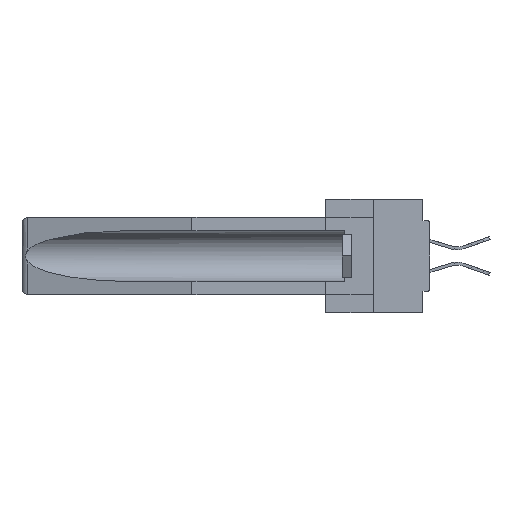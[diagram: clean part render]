
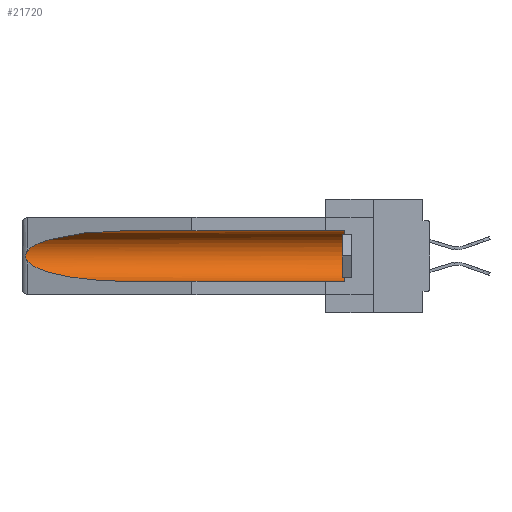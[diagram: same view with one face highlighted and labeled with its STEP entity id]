
A CAD part, left-side view. The second image highlights one B-rep face of the part: STEP entity #21720.
In plain terms, the highlighted cylindrical face has radius 2.857 mm (diameter 5.715 mm), a partial arc.
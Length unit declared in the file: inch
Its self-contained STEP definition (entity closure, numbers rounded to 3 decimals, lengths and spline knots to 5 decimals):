
#27 = EDGE_CURVE ( 'NONE', #23490, #26655, #21769, .T. ) ;
#66 = CARTESIAN_POINT ( 'NONE',  ( 0.2675, 1.53308, -0.16763 ) ) ;
#381 = EDGE_LOOP ( 'NONE', ( #35002, #39673, #11307, #32883, #12412, #17191 ) ) ;
#655 = EDGE_CURVE ( 'NONE', #15124, #21723, #30816, .T. ) ;
#1708 = AXIS2_PLACEMENT_3D ( 'NONE', #29008, #10646, #13699 ) ;
#2555 = CARTESIAN_POINT ( 'NONE',  ( 0.155, -0.30754, -0.059 ) ) ;
#6058 = CARTESIAN_POINT ( 'NONE',  ( 0.26654, 1.53092, -0.15636 ) ) ;
#8360 = CARTESIAN_POINT ( 'NONE',  ( 0.155, 0.126, -0.1715 ) ) ;
#8729 = CARTESIAN_POINT ( 'NONE',  ( 0.26537, 1.52718, -0.19328 ) ) ;
#8858 = CARTESIAN_POINT ( 'NONE',  ( 0.26597, 1.5296, -0.19026 ) ) ;
#8891 = CARTESIAN_POINT ( 'NONE',  ( 0.26537, 1.52718, -0.14972 ) ) ;
#9084 = VECTOR ( 'NONE', #39557, 39.37008 ) ;
#9232 = CARTESIAN_POINT ( 'NONE',  ( 0.21114, 1.30732, -0.059 ) ) ;
#10646 = DIRECTION ( 'NONE',  ( 0., 1., 0. ) ) ;
#11240 = VERTEX_POINT ( 'NONE', #8891 ) ;
#11307 = ORIENTED_EDGE ( 'NONE', *, *, #27, .T. ) ;
#12412 = ORIENTED_EDGE ( 'NONE', *, *, #655, .T. ) ;
#13699 = DIRECTION ( 'NONE',  ( 0., 0., 1. ) ) ;
#14834 = LINE ( 'NONE', #2555, #9084 ) ;
#15124 = VERTEX_POINT ( 'NONE', #22785 ) ;
#15191 = CARTESIAN_POINT ( 'NONE',  ( 0.25451, 1.48313, -0.24835 ) ) ;
#15250 = CARTESIAN_POINT ( 'NONE',  ( 0.26537, 1.52718, -0.19328 ) ) ;
#15531 = EDGE_CURVE ( 'NONE', #38226, #11240, #17136, .T. ) ;
#16659 = LINE ( 'NONE', #20119, #23309 ) ;
#17136 =( BOUNDED_CURVE ( )  B_SPLINE_CURVE ( 3, ( #36524, #9232, #37329, #37182 ),
 .UNSPECIFIED., .F., .F. ) 
 B_SPLINE_CURVE_WITH_KNOTS ( ( 4, 4 ),
 ( 4.71239, 6.08839 ),
 .UNSPECIFIED. ) 
 CURVE ( )  GEOMETRIC_REPRESENTATION_ITEM ( )  RATIONAL_B_SPLINE_CURVE ( ( 1., 0.848, 0.848, 1. ) ) 
 REPRESENTATION_ITEM ( '' )  );
#17191 = ORIENTED_EDGE ( 'NONE', *, *, #30240, .T. ) ;
#19035 = AXIS2_PLACEMENT_3D ( 'NONE', #8360, #28179, #21498 ) ;
#19259 = B_SPLINE_CURVE_WITH_KNOTS ( 'NONE', 3,
 ( #27321, #24142, #6058, #33700, #66, #27057, #36795, #34310, #8858, #8729 ),
 .UNSPECIFIED., .F., .F.,
 ( 4, 2, 2, 2, 4 ),
 ( 0., 0.00029, 0.00058, 0.00087, 0.00117 ),
 .UNSPECIFIED. ) ;
#20119 = CARTESIAN_POINT ( 'NONE',  ( 0.155, -0.30754, -0.284 ) ) ;
#21498 = DIRECTION ( 'NONE',  ( 0., 0., 1. ) ) ;
#21720 = ADVANCED_FACE ( 'NONE', ( #34038 ), #39353, .F. ) ;
#21723 = VERTEX_POINT ( 'NONE', #28746 ) ;
#21769 =( BOUNDED_CURVE ( )  B_SPLINE_CURVE ( 3, ( #27908, #15191, #27367, #30508 ),
 .UNSPECIFIED., .F., .F. ) 
 B_SPLINE_CURVE_WITH_KNOTS ( ( 4, 4 ),
 ( 0.1948, 1.5708 ),
 .UNSPECIFIED. ) 
 CURVE ( )  GEOMETRIC_REPRESENTATION_ITEM ( )  RATIONAL_B_SPLINE_CURVE ( ( 1., 0.848, 0.848, 1. ) ) 
 REPRESENTATION_ITEM ( '' )  );
#22646 = EDGE_CURVE ( 'NONE', #15124, #26655, #16659, .T. ) ;
#22785 = CARTESIAN_POINT ( 'NONE',  ( 0.155, 0.126, -0.284 ) ) ;
#23309 = VECTOR ( 'NONE', #38339, 39.37008 ) ;
#23490 = VERTEX_POINT ( 'NONE', #15250 ) ;
#24142 = CARTESIAN_POINT ( 'NONE',  ( 0.26597, 1.52961, -0.15275 ) ) ;
#26655 = VERTEX_POINT ( 'NONE', #26999 ) ;
#26952 = EDGE_CURVE ( 'NONE', #11240, #23490, #19259, .T. ) ;
#26999 = CARTESIAN_POINT ( 'NONE',  ( 0.155, 1.07973, -0.284 ) ) ;
#27057 = CARTESIAN_POINT ( 'NONE',  ( 0.2675, 1.53308, -0.17534 ) ) ;
#27321 = CARTESIAN_POINT ( 'NONE',  ( 0.26537, 1.52718, -0.14972 ) ) ;
#27367 = CARTESIAN_POINT ( 'NONE',  ( 0.21114, 1.30732, -0.284 ) ) ;
#27908 = CARTESIAN_POINT ( 'NONE',  ( 0.26537, 1.52718, -0.19328 ) ) ;
#28179 = DIRECTION ( 'NONE',  ( 0., -1., 0. ) ) ;
#28746 = CARTESIAN_POINT ( 'NONE',  ( 0.155, 0.126, -0.059 ) ) ;
#29008 = CARTESIAN_POINT ( 'NONE',  ( 0.155, -0.30754, -0.1715 ) ) ;
#30240 = EDGE_CURVE ( 'NONE', #21723, #38226, #14834, .T. ) ;
#30508 = CARTESIAN_POINT ( 'NONE',  ( 0.155, 1.07973, -0.284 ) ) ;
#30816 = CIRCLE ( 'NONE', #19035, 0.1125 ) ;
#32883 = ORIENTED_EDGE ( 'NONE', *, *, #22646, .F. ) ;
#33700 = CARTESIAN_POINT ( 'NONE',  ( 0.2673, 1.5327, -0.16383 ) ) ;
#34038 = FACE_OUTER_BOUND ( 'NONE', #381, .T. ) ;
#34310 = CARTESIAN_POINT ( 'NONE',  ( 0.26655, 1.53094, -0.18657 ) ) ;
#34535 = CARTESIAN_POINT ( 'NONE',  ( 0.155, 1.07973, -0.059 ) ) ;
#35002 = ORIENTED_EDGE ( 'NONE', *, *, #15531, .T. ) ;
#36524 = CARTESIAN_POINT ( 'NONE',  ( 0.155, 1.07973, -0.059 ) ) ;
#36795 = CARTESIAN_POINT ( 'NONE',  ( 0.2673, 1.53269, -0.17917 ) ) ;
#37182 = CARTESIAN_POINT ( 'NONE',  ( 0.26537, 1.52718, -0.14972 ) ) ;
#37329 = CARTESIAN_POINT ( 'NONE',  ( 0.25451, 1.48313, -0.09465 ) ) ;
#38226 = VERTEX_POINT ( 'NONE', #34535 ) ;
#38339 = DIRECTION ( 'NONE',  ( 0., 1., 0. ) ) ;
#39353 = CYLINDRICAL_SURFACE ( 'NONE', #1708, 0.1125 ) ;
#39557 = DIRECTION ( 'NONE',  ( 0., 1., 0. ) ) ;
#39673 = ORIENTED_EDGE ( 'NONE', *, *, #26952, .T. ) ;
